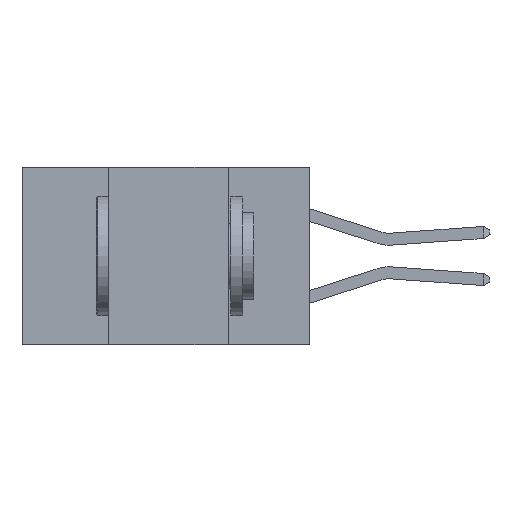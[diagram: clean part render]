
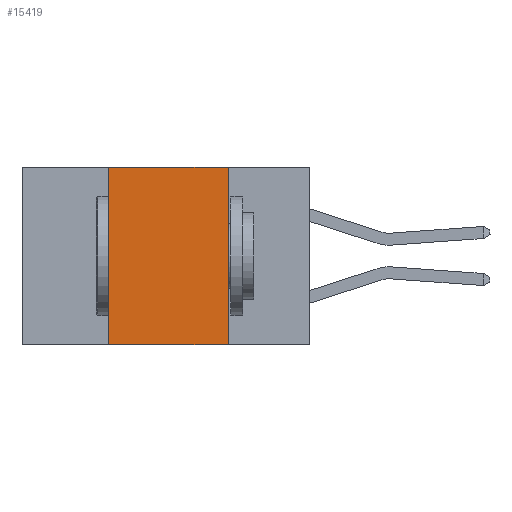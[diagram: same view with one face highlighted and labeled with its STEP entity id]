
A CAD part, left-side view. The second image highlights one B-rep face of the part: STEP entity #15419.
In plain terms, the highlighted planar face has unit normal (-1, 0, 0).
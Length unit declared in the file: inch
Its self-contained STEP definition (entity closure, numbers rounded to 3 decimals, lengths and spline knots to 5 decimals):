
#253 = ORIENTED_EDGE ( 'NONE', *, *, #13127, .T. ) ;
#724 = LINE ( 'NONE', #9030, #17022 ) ;
#1032 = CARTESIAN_POINT ( 'NONE',  ( 0., 0.42, 0. ) ) ;
#1413 = VERTEX_POINT ( 'NONE', #5740 ) ;
#1522 = CARTESIAN_POINT ( 'NONE',  ( 0., 0.17, -0.37 ) ) ;
#1556 = ORIENTED_EDGE ( 'NONE', *, *, #2844, .F. ) ;
#2232 = EDGE_CURVE ( 'NONE', #9053, #1413, #2519, .T. ) ;
#2519 = LINE ( 'NONE', #8995, #9186 ) ;
#2844 = EDGE_CURVE ( 'NONE', #1413, #14793, #10608, .T. ) ;
#3388 = DIRECTION ( 'NONE',  ( 0., -1., 0. ) ) ;
#4845 = VECTOR ( 'NONE', #5128, 39.37008 ) ;
#4971 = CARTESIAN_POINT ( 'NONE',  ( 0., 0.17, -0.37 ) ) ;
#5128 = DIRECTION ( 'NONE',  ( 0., 0., -1. ) ) ;
#5740 = CARTESIAN_POINT ( 'NONE',  ( 0., 0.17, 0. ) ) ;
#6656 = ORIENTED_EDGE ( 'NONE', *, *, #7078, .F. ) ;
#7078 = EDGE_CURVE ( 'NONE', #8015, #9053, #724, .T. ) ;
#7686 = DIRECTION ( 'NONE',  ( 1., 0., 0. ) ) ;
#8015 = VERTEX_POINT ( 'NONE', #13611 ) ;
#8995 = CARTESIAN_POINT ( 'NONE',  ( 0., 0.6, 0. ) ) ;
#9030 = CARTESIAN_POINT ( 'NONE',  ( 0., 0.42, -0.37 ) ) ;
#9035 = VECTOR ( 'NONE', #3388, 39.37008 ) ;
#9053 = VERTEX_POINT ( 'NONE', #1032 ) ;
#9186 = VECTOR ( 'NONE', #16886, 39.37008 ) ;
#9538 = FACE_OUTER_BOUND ( 'NONE', #13174, .T. ) ;
#10338 = DIRECTION ( 'NONE',  ( 0., 0., 1. ) ) ;
#10401 = AXIS2_PLACEMENT_3D ( 'NONE', #15451, #7686, #16751 ) ;
#10608 = LINE ( 'NONE', #4971, #4845 ) ;
#11695 = LINE ( 'NONE', #12606, #9035 ) ;
#12606 = CARTESIAN_POINT ( 'NONE',  ( 0., 0.6, -0.37 ) ) ;
#13127 = EDGE_CURVE ( 'NONE', #8015, #14793, #11695, .T. ) ;
#13174 = EDGE_LOOP ( 'NONE', ( #1556, #16195, #6656, #253 ) ) ;
#13611 = CARTESIAN_POINT ( 'NONE',  ( 0., 0.42, -0.37 ) ) ;
#14793 = VERTEX_POINT ( 'NONE', #1522 ) ;
#15393 = PLANE ( 'NONE',  #10401 ) ;
#15419 = ADVANCED_FACE ( 'NONE', ( #9538 ), #15393, .F. ) ;
#15451 = CARTESIAN_POINT ( 'NONE',  ( 0., 0.6, 0. ) ) ;
#16195 = ORIENTED_EDGE ( 'NONE', *, *, #2232, .F. ) ;
#16751 = DIRECTION ( 'NONE',  ( 0., 0., -1. ) ) ;
#16886 = DIRECTION ( 'NONE',  ( 0., -1., 0. ) ) ;
#17022 = VECTOR ( 'NONE', #10338, 39.37008 ) ;
